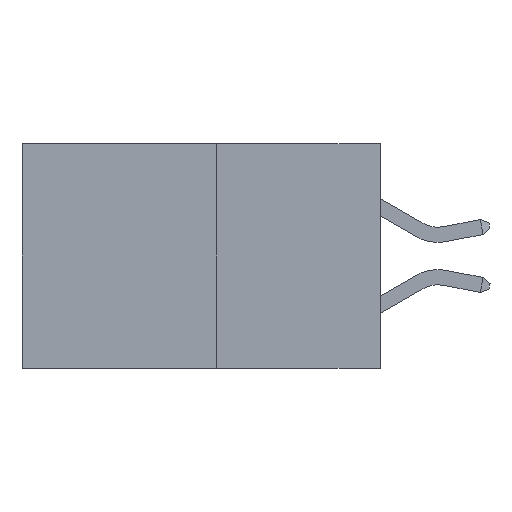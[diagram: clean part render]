
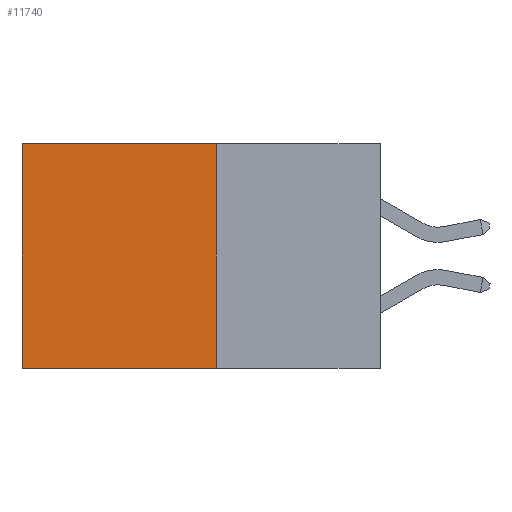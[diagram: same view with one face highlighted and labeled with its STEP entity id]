
A CAD part, left-side view. The second image highlights one B-rep face of the part: STEP entity #11740.
In plain terms, the highlighted planar face has unit normal (-1, 0, 0).
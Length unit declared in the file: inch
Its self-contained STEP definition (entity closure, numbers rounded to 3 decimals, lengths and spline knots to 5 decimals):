
#57 = ORIENTED_EDGE ( 'NONE', *, *, #1286, .T. ) ;
#405 = EDGE_CURVE ( 'NONE', #14818, #15056, #5245, .T. ) ;
#1286 = EDGE_CURVE ( 'NONE', #14892, #13510, #1369, .T. ) ;
#1369 = LINE ( 'NONE', #4947, #16638 ) ;
#1959 = CARTESIAN_POINT ( 'NONE',  ( 0.277, 0.27, -0.37 ) ) ;
#2475 = DIRECTION ( 'NONE',  ( 0., 1., 0. ) ) ;
#3438 = CARTESIAN_POINT ( 'NONE',  ( 0.277, 0.27, -0.37 ) ) ;
#3939 = VECTOR ( 'NONE', #5480, 39.37008 ) ;
#4278 = EDGE_LOOP ( 'NONE', ( #13615, #10691, #14496, #57 ) ) ;
#4396 = LINE ( 'NONE', #5599, #3939 ) ;
#4875 = DIRECTION ( 'NONE',  ( 1., 0., 0. ) ) ;
#4947 = CARTESIAN_POINT ( 'NONE',  ( 0.277, 0.27, 0. ) ) ;
#5245 = LINE ( 'NONE', #1959, #12003 ) ;
#5480 = DIRECTION ( 'NONE',  ( 0., 0., -1. ) ) ;
#5599 = CARTESIAN_POINT ( 'NONE',  ( 0.277, 0.27, -0.37 ) ) ;
#5659 = FACE_OUTER_BOUND ( 'NONE', #4278, .T. ) ;
#5803 = CARTESIAN_POINT ( 'NONE',  ( 0.277, 0.27, -0.37 ) ) ;
#7658 = DIRECTION ( 'NONE',  ( 0., 0., -1. ) ) ;
#7899 = EDGE_CURVE ( 'NONE', #14892, #14818, #4396, .T. ) ;
#8537 = AXIS2_PLACEMENT_3D ( 'NONE', #3438, #4875, #14933 ) ;
#10691 = ORIENTED_EDGE ( 'NONE', *, *, #405, .F. ) ;
#11371 = CARTESIAN_POINT ( 'NONE',  ( 0.277, 0.59, 0. ) ) ;
#11648 = CARTESIAN_POINT ( 'NONE',  ( 0.277, 0.27, 0. ) ) ;
#11740 = ADVANCED_FACE ( 'NONE', ( #5659 ), #13501, .F. ) ;
#12003 = VECTOR ( 'NONE', #2475, 39.37008 ) ;
#12819 = LINE ( 'NONE', #16249, #16585 ) ;
#13501 = PLANE ( 'NONE',  #8537 ) ;
#13510 = VERTEX_POINT ( 'NONE', #11371 ) ;
#13615 = ORIENTED_EDGE ( 'NONE', *, *, #18130, .T. ) ;
#14496 = ORIENTED_EDGE ( 'NONE', *, *, #7899, .F. ) ;
#14818 = VERTEX_POINT ( 'NONE', #5803 ) ;
#14892 = VERTEX_POINT ( 'NONE', #11648 ) ;
#14933 = DIRECTION ( 'NONE',  ( 0., 0., -1. ) ) ;
#15056 = VERTEX_POINT ( 'NONE', #17633 ) ;
#16074 = DIRECTION ( 'NONE',  ( 0., 1., 0. ) ) ;
#16249 = CARTESIAN_POINT ( 'NONE',  ( 0.277, 0.59, -0.37 ) ) ;
#16585 = VECTOR ( 'NONE', #7658, 39.37008 ) ;
#16638 = VECTOR ( 'NONE', #16074, 39.37008 ) ;
#17633 = CARTESIAN_POINT ( 'NONE',  ( 0.277, 0.59, -0.37 ) ) ;
#18130 = EDGE_CURVE ( 'NONE', #13510, #15056, #12819, .T. ) ;
